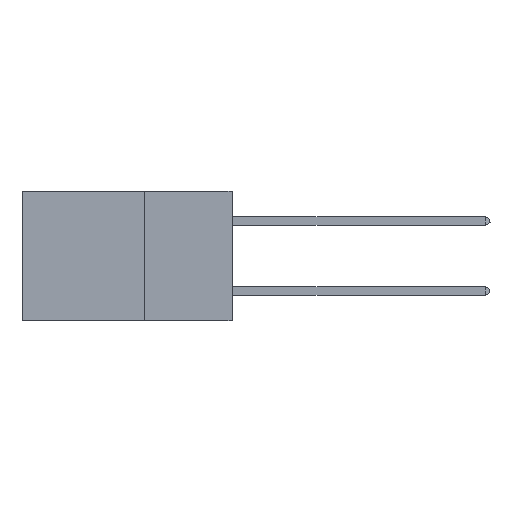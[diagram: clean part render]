
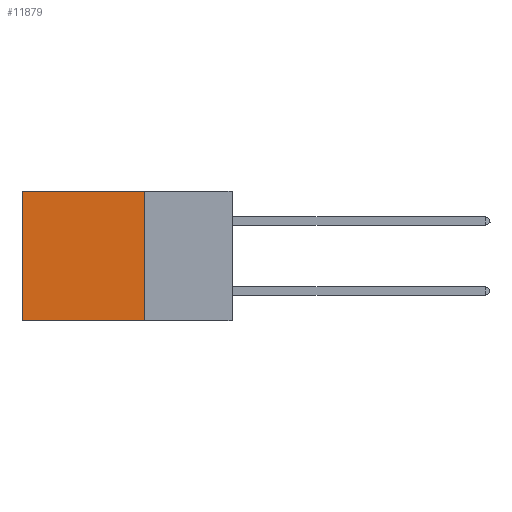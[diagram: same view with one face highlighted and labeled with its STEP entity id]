
A CAD part, left-side view. The second image highlights one B-rep face of the part: STEP entity #11879.
In plain terms, the highlighted planar face has unit normal (-1, 0, 0).
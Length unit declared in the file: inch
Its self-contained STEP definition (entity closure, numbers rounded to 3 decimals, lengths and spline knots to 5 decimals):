
#199 = DIRECTION ( 'NONE',  ( 1., 0., 0. ) ) ;
#1149 = LINE ( 'NONE', #5184, #21209 ) ;
#3102 = EDGE_CURVE ( 'NONE', #13758, #9348, #16223, .T. ) ;
#3965 = PLANE ( 'NONE',  #19697 ) ;
#4486 = DIRECTION ( 'NONE',  ( 0., 0., -1. ) ) ;
#4816 = CARTESIAN_POINT ( 'NONE',  ( 0.2875, 0.25, 0. ) ) ;
#4956 = EDGE_CURVE ( 'NONE', #9348, #19453, #1149, .T. ) ;
#5184 = CARTESIAN_POINT ( 'NONE',  ( 0.2875, 0.25, -0.37 ) ) ;
#5486 = FACE_OUTER_BOUND ( 'NONE', #14161, .T. ) ;
#6030 = CARTESIAN_POINT ( 'NONE',  ( 0.2875, 0.25, 0. ) ) ;
#7240 = VECTOR ( 'NONE', #9398, 39.37008 ) ;
#7567 = CARTESIAN_POINT ( 'NONE',  ( 0.2875, 0.25, -0.37 ) ) ;
#7588 = ORIENTED_EDGE ( 'NONE', *, *, #3102, .F. ) ;
#8241 = VECTOR ( 'NONE', #14294, 39.37008 ) ;
#9348 = VERTEX_POINT ( 'NONE', #7567 ) ;
#9398 = DIRECTION ( 'NONE',  ( 0., 0., -1. ) ) ;
#10858 = VERTEX_POINT ( 'NONE', #19095 ) ;
#11879 = ADVANCED_FACE ( 'NONE', ( #5486 ), #3965, .F. ) ;
#11972 = CARTESIAN_POINT ( 'NONE',  ( 0.2875, 0.25, 0. ) ) ;
#12426 = VECTOR ( 'NONE', #15382, 39.37008 ) ;
#13255 = EDGE_CURVE ( 'NONE', #13758, #10858, #24448, .T. ) ;
#13617 = EDGE_CURVE ( 'NONE', #10858, #19453, #26352, .T. ) ;
#13676 = DIRECTION ( 'NONE',  ( 0., 1., 0. ) ) ;
#13758 = VERTEX_POINT ( 'NONE', #11972 ) ;
#14161 = EDGE_LOOP ( 'NONE', ( #25309, #25805, #7588, #18522 ) ) ;
#14294 = DIRECTION ( 'NONE',  ( 0., 1., 0. ) ) ;
#15382 = DIRECTION ( 'NONE',  ( 0., 0., -1. ) ) ;
#16223 = LINE ( 'NONE', #4816, #12426 ) ;
#17557 = CARTESIAN_POINT ( 'NONE',  ( 0.2875, 0.6, 0. ) ) ;
#18293 = CARTESIAN_POINT ( 'NONE',  ( 0.2875, 0.25, 0. ) ) ;
#18522 = ORIENTED_EDGE ( 'NONE', *, *, #13255, .T. ) ;
#19095 = CARTESIAN_POINT ( 'NONE',  ( 0.2875, 0.6, 0. ) ) ;
#19453 = VERTEX_POINT ( 'NONE', #24262 ) ;
#19697 = AXIS2_PLACEMENT_3D ( 'NONE', #6030, #199, #4486 ) ;
#21209 = VECTOR ( 'NONE', #13676, 39.37008 ) ;
#24262 = CARTESIAN_POINT ( 'NONE',  ( 0.2875, 0.6, -0.37 ) ) ;
#24448 = LINE ( 'NONE', #18293, #8241 ) ;
#25309 = ORIENTED_EDGE ( 'NONE', *, *, #13617, .T. ) ;
#25805 = ORIENTED_EDGE ( 'NONE', *, *, #4956, .F. ) ;
#26352 = LINE ( 'NONE', #17557, #7240 ) ;
